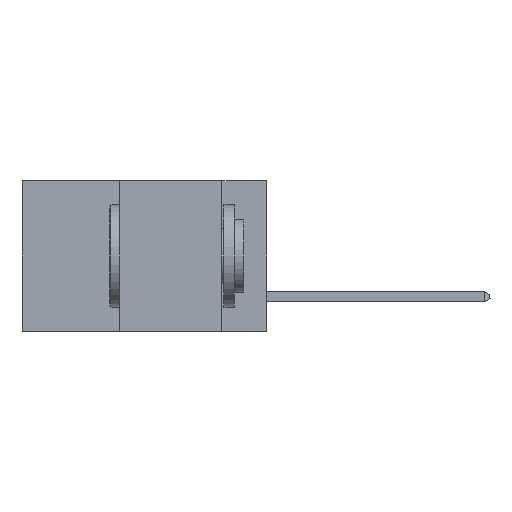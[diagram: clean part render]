
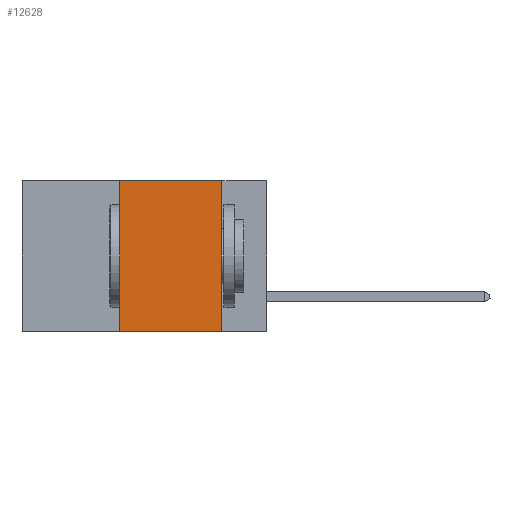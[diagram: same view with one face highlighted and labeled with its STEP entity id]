
A CAD part, left-side view. The second image highlights one B-rep face of the part: STEP entity #12628.
In plain terms, the highlighted planar face has unit normal (-1, 0, 0).
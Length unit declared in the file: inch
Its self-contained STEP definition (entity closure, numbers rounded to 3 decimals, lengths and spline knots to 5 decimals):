
#289 = PLANE ( 'NONE',  #526 ) ;
#526 = AXIS2_PLACEMENT_3D ( 'NONE', #1620, #5603, #6898 ) ;
#653 = CARTESIAN_POINT ( 'NONE',  ( 0., 0.36, 0. ) ) ;
#843 = VECTOR ( 'NONE', #3025, 39.37008 ) ;
#1190 = VERTEX_POINT ( 'NONE', #16549 ) ;
#1620 = CARTESIAN_POINT ( 'NONE',  ( 0., 0.6, 0. ) ) ;
#2090 = CARTESIAN_POINT ( 'NONE',  ( 0., 0.11, 0. ) ) ;
#2534 = VERTEX_POINT ( 'NONE', #5872 ) ;
#2618 = ORIENTED_EDGE ( 'NONE', *, *, #11736, .F. ) ;
#3025 = DIRECTION ( 'NONE',  ( 0., -1., 0. ) ) ;
#3275 = VERTEX_POINT ( 'NONE', #2090 ) ;
#4134 = VERTEX_POINT ( 'NONE', #6266 ) ;
#4412 = CARTESIAN_POINT ( 'NONE',  ( 0., 0.6, -0.37 ) ) ;
#4643 = EDGE_LOOP ( 'NONE', ( #11965, #13656, #2618, #11864 ) ) ;
#4671 = EDGE_CURVE ( 'NONE', #4134, #2534, #6859, .T. ) ;
#5603 = DIRECTION ( 'NONE',  ( 1., 0., 0. ) ) ;
#5872 = CARTESIAN_POINT ( 'NONE',  ( 0., 0.11, -0.37 ) ) ;
#6266 = CARTESIAN_POINT ( 'NONE',  ( 0., 0.36, -0.37 ) ) ;
#6859 = LINE ( 'NONE', #4412, #11802 ) ;
#6867 = EDGE_CURVE ( 'NONE', #1190, #3275, #10305, .T. ) ;
#6898 = DIRECTION ( 'NONE',  ( 0., 0., -1. ) ) ;
#7126 = DIRECTION ( 'NONE',  ( 0., -1., 0. ) ) ;
#7835 = EDGE_CURVE ( 'NONE', #3275, #2534, #15906, .T. ) ;
#8858 = VECTOR ( 'NONE', #13635, 39.37008 ) ;
#9518 = VECTOR ( 'NONE', #11327, 39.37008 ) ;
#10305 = LINE ( 'NONE', #15902, #843 ) ;
#11327 = DIRECTION ( 'NONE',  ( 0., 0., -1. ) ) ;
#11736 = EDGE_CURVE ( 'NONE', #4134, #1190, #14751, .T. ) ;
#11802 = VECTOR ( 'NONE', #7126, 39.37008 ) ;
#11864 = ORIENTED_EDGE ( 'NONE', *, *, #4671, .T. ) ;
#11965 = ORIENTED_EDGE ( 'NONE', *, *, #7835, .F. ) ;
#12628 = ADVANCED_FACE ( 'NONE', ( #14713 ), #289, .F. ) ;
#13635 = DIRECTION ( 'NONE',  ( 0., 0., 1. ) ) ;
#13656 = ORIENTED_EDGE ( 'NONE', *, *, #6867, .F. ) ;
#14713 = FACE_OUTER_BOUND ( 'NONE', #4643, .T. ) ;
#14751 = LINE ( 'NONE', #653, #8858 ) ;
#15167 = CARTESIAN_POINT ( 'NONE',  ( 0., 0.11, 0. ) ) ;
#15902 = CARTESIAN_POINT ( 'NONE',  ( 0., 0.6, 0. ) ) ;
#15906 = LINE ( 'NONE', #15167, #9518 ) ;
#16549 = CARTESIAN_POINT ( 'NONE',  ( 0., 0.36, 0. ) ) ;
